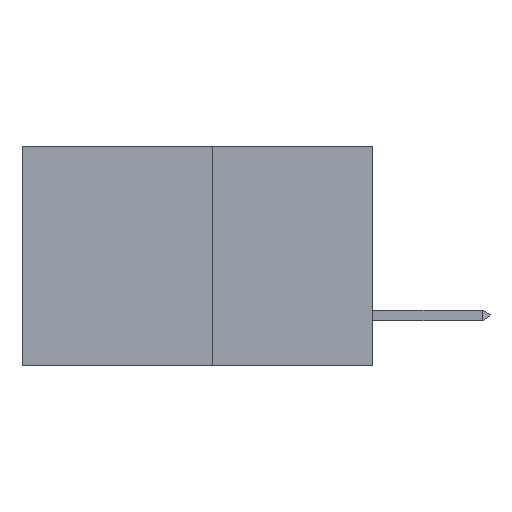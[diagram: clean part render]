
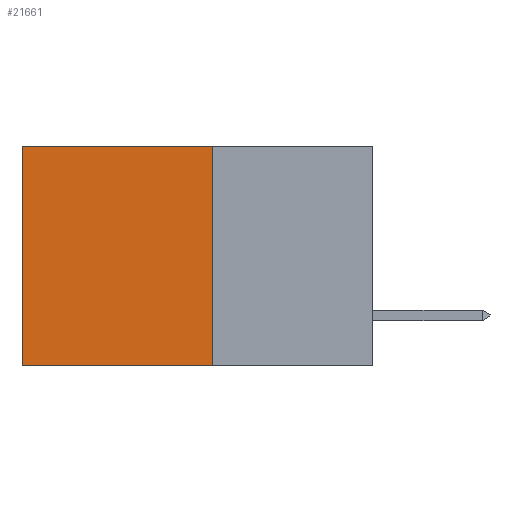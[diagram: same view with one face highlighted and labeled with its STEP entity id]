
A CAD part, left-side view. The second image highlights one B-rep face of the part: STEP entity #21661.
In plain terms, the highlighted planar face has unit normal (-1, 0, 0).
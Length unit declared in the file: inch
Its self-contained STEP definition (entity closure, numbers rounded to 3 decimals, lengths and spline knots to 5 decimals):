
#1482 = VERTEX_POINT ( 'NONE', #7008 ) ;
#2708 = LINE ( 'NONE', #19332, #11861 ) ;
#3404 = EDGE_CURVE ( 'NONE', #11870, #10008, #19228, .T. ) ;
#3905 = EDGE_CURVE ( 'NONE', #10008, #4670, #2708, .T. ) ;
#4670 = VERTEX_POINT ( 'NONE', #22090 ) ;
#5141 = CARTESIAN_POINT ( 'NONE',  ( 0.277, 0.59, 0. ) ) ;
#6107 = FACE_OUTER_BOUND ( 'NONE', #13518, .T. ) ;
#7008 = CARTESIAN_POINT ( 'NONE',  ( 0.277, 0.27, -0.37 ) ) ;
#7127 = CARTESIAN_POINT ( 'NONE',  ( 0.277, 0.27, -0.37 ) ) ;
#7991 = CARTESIAN_POINT ( 'NONE',  ( 0.277, 0.27, 0. ) ) ;
#8712 = VECTOR ( 'NONE', #18467, 39.37008 ) ;
#8985 = DIRECTION ( 'NONE',  ( 0., 0., -1. ) ) ;
#9154 = EDGE_CURVE ( 'NONE', #1482, #4670, #9833, .T. ) ;
#9248 = ORIENTED_EDGE ( 'NONE', *, *, #3404, .T. ) ;
#9833 = LINE ( 'NONE', #19391, #19769 ) ;
#10008 = VERTEX_POINT ( 'NONE', #5141 ) ;
#10417 = CARTESIAN_POINT ( 'NONE',  ( 0.277, 0.27, -0.37 ) ) ;
#11861 = VECTOR ( 'NONE', #19411, 39.37008 ) ;
#11870 = VERTEX_POINT ( 'NONE', #7991 ) ;
#12139 = LINE ( 'NONE', #7127, #15958 ) ;
#12293 = DIRECTION ( 'NONE',  ( 0., 0., -1. ) ) ;
#13518 = EDGE_LOOP ( 'NONE', ( #21093, #13842, #17450, #9248 ) ) ;
#13842 = ORIENTED_EDGE ( 'NONE', *, *, #9154, .F. ) ;
#15958 = VECTOR ( 'NONE', #8985, 39.37008 ) ;
#16610 = AXIS2_PLACEMENT_3D ( 'NONE', #10417, #23444, #12293 ) ;
#17450 = ORIENTED_EDGE ( 'NONE', *, *, #22528, .F. ) ;
#17768 = PLANE ( 'NONE',  #16610 ) ;
#18467 = DIRECTION ( 'NONE',  ( 0., 1., 0. ) ) ;
#18638 = CARTESIAN_POINT ( 'NONE',  ( 0.277, 0.27, 0. ) ) ;
#19228 = LINE ( 'NONE', #18638, #8712 ) ;
#19314 = DIRECTION ( 'NONE',  ( 0., 1., 0. ) ) ;
#19332 = CARTESIAN_POINT ( 'NONE',  ( 0.277, 0.59, -0.37 ) ) ;
#19391 = CARTESIAN_POINT ( 'NONE',  ( 0.277, 0.27, -0.37 ) ) ;
#19411 = DIRECTION ( 'NONE',  ( 0., 0., -1. ) ) ;
#19769 = VECTOR ( 'NONE', #19314, 39.37008 ) ;
#21093 = ORIENTED_EDGE ( 'NONE', *, *, #3905, .T. ) ;
#21661 = ADVANCED_FACE ( 'NONE', ( #6107 ), #17768, .F. ) ;
#22090 = CARTESIAN_POINT ( 'NONE',  ( 0.277, 0.59, -0.37 ) ) ;
#22528 = EDGE_CURVE ( 'NONE', #11870, #1482, #12139, .T. ) ;
#23444 = DIRECTION ( 'NONE',  ( 1., 0., 0. ) ) ;
